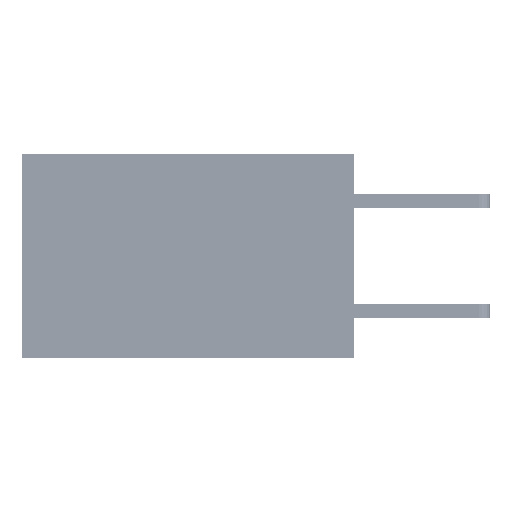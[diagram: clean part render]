
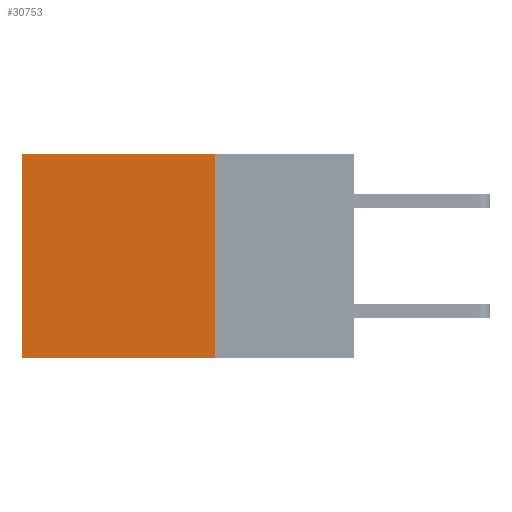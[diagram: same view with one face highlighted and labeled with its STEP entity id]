
A CAD part, left-side view. The second image highlights one B-rep face of the part: STEP entity #30753.
In plain terms, the highlighted planar face has unit normal (-1, 0, 0).
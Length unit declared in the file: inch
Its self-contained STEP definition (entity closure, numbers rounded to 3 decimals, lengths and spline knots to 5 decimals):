
#1318 = AXIS2_PLACEMENT_3D ( 'NONE', #3343, #6898, #31743 ) ;
#3070 = VERTEX_POINT ( 'NONE', #45288 ) ;
#3343 = CARTESIAN_POINT ( 'NONE',  ( 0.2875, 0.25, 0. ) ) ;
#3498 = FACE_OUTER_BOUND ( 'NONE', #23472, .T. ) ;
#4276 = ORIENTED_EDGE ( 'NONE', *, *, #34998, .F. ) ;
#4966 = VECTOR ( 'NONE', #36160, 39.37008 ) ;
#6898 = DIRECTION ( 'NONE',  ( 1., 0., 0. ) ) ;
#6945 = CARTESIAN_POINT ( 'NONE',  ( 0.2875, 0.6, 0. ) ) ;
#8367 = EDGE_CURVE ( 'NONE', #3070, #17543, #12072, .T. ) ;
#8404 = CARTESIAN_POINT ( 'NONE',  ( 0.2875, 0.6, 0. ) ) ;
#10499 = LINE ( 'NONE', #22776, #18858 ) ;
#10732 = CARTESIAN_POINT ( 'NONE',  ( 0.2875, 0.25, 0. ) ) ;
#12072 = LINE ( 'NONE', #10732, #39230 ) ;
#12098 = DIRECTION ( 'NONE',  ( 0., 1., 0. ) ) ;
#13191 = VERTEX_POINT ( 'NONE', #18547 ) ;
#14054 = CARTESIAN_POINT ( 'NONE',  ( 0.2875, 0.25, -0.37 ) ) ;
#17171 = ORIENTED_EDGE ( 'NONE', *, *, #8367, .T. ) ;
#17543 = VERTEX_POINT ( 'NONE', #8404 ) ;
#18547 = CARTESIAN_POINT ( 'NONE',  ( 0.2875, 0.6, -0.37 ) ) ;
#18858 = VECTOR ( 'NONE', #12098, 39.37008 ) ;
#22776 = CARTESIAN_POINT ( 'NONE',  ( 0.2875, 0.25, -0.37 ) ) ;
#23472 = EDGE_LOOP ( 'NONE', ( #24537, #4276, #23973, #17171 ) ) ;
#23771 = EDGE_CURVE ( 'NONE', #17543, #13191, #42797, .T. ) ;
#23973 = ORIENTED_EDGE ( 'NONE', *, *, #24602, .F. ) ;
#24537 = ORIENTED_EDGE ( 'NONE', *, *, #23771, .T. ) ;
#24584 = PLANE ( 'NONE',  #1318 ) ;
#24602 = EDGE_CURVE ( 'NONE', #3070, #29101, #42713, .T. ) ;
#29101 = VERTEX_POINT ( 'NONE', #14054 ) ;
#30753 = ADVANCED_FACE ( 'NONE', ( #3498 ), #24584, .F. ) ;
#31743 = DIRECTION ( 'NONE',  ( 0., 0., -1. ) ) ;
#32639 = CARTESIAN_POINT ( 'NONE',  ( 0.2875, 0.25, 0. ) ) ;
#34496 = VECTOR ( 'NONE', #35346, 39.37008 ) ;
#34998 = EDGE_CURVE ( 'NONE', #29101, #13191, #10499, .T. ) ;
#35346 = DIRECTION ( 'NONE',  ( 0., 0., -1. ) ) ;
#36160 = DIRECTION ( 'NONE',  ( 0., 0., -1. ) ) ;
#39230 = VECTOR ( 'NONE', #44793, 39.37008 ) ;
#42713 = LINE ( 'NONE', #32639, #4966 ) ;
#42797 = LINE ( 'NONE', #6945, #34496 ) ;
#44793 = DIRECTION ( 'NONE',  ( 0., 1., 0. ) ) ;
#45288 = CARTESIAN_POINT ( 'NONE',  ( 0.2875, 0.25, 0. ) ) ;
